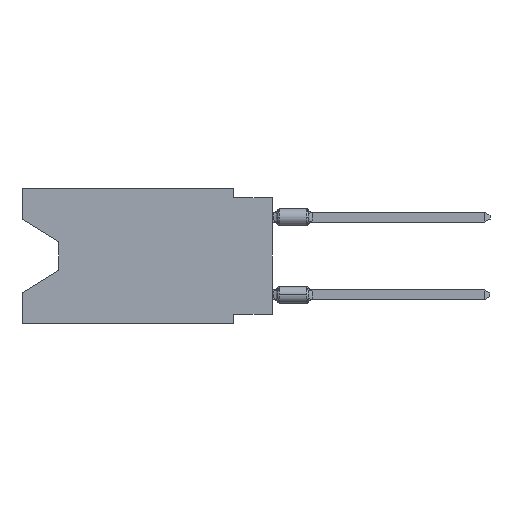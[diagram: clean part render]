
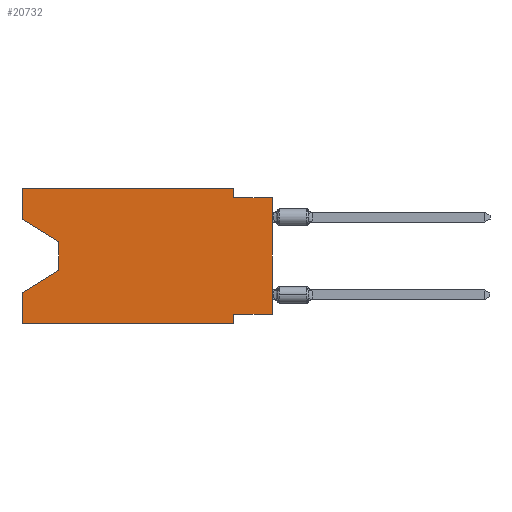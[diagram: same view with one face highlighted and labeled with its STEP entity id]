
A CAD part, left-side view. The second image highlights one B-rep face of the part: STEP entity #20732.
In plain terms, the highlighted planar face has unit normal (-1, 0, 0).
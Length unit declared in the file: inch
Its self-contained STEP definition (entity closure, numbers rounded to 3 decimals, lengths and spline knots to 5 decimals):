
#226 = CARTESIAN_POINT ( 'NONE',  ( 0., 0.1, -0.35 ) ) ;
#318 = LINE ( 'NONE', #9425, #13869 ) ;
#330 = LINE ( 'NONE', #23256, #6526 ) ;
#856 = EDGE_CURVE ( 'NONE', #12084, #20970, #318, .T. ) ;
#1134 = ORIENTED_EDGE ( 'NONE', *, *, #16072, .T. ) ;
#1196 = VECTOR ( 'NONE', #19495, 39.37008 ) ;
#1309 = CARTESIAN_POINT ( 'NONE',  ( 0., 0.55, -0.212 ) ) ;
#1514 = VECTOR ( 'NONE', #25624, 39.37008 ) ;
#1597 = CARTESIAN_POINT ( 'NONE',  ( 0., 0.55, -0.138 ) ) ;
#2020 = ORIENTED_EDGE ( 'NONE', *, *, #13922, .F. ) ;
#2694 = VECTOR ( 'NONE', #11086, 39.37008 ) ;
#2891 = DIRECTION ( 'NONE',  ( 0., 0., 1. ) ) ;
#3900 = VECTOR ( 'NONE', #18165, 39.37008 ) ;
#4437 = ORIENTED_EDGE ( 'NONE', *, *, #6137, .T. ) ;
#4848 = LINE ( 'NONE', #226, #22585 ) ;
#4886 = VERTEX_POINT ( 'NONE', #15136 ) ;
#5047 = EDGE_CURVE ( 'NONE', #11551, #13880, #15594, .T. ) ;
#5419 = CARTESIAN_POINT ( 'NONE',  ( 0., 0.645, 0. ) ) ;
#5496 = EDGE_CURVE ( 'NONE', #18941, #4886, #27695, .T. ) ;
#6137 = EDGE_CURVE ( 'NONE', #6393, #21999, #13539, .T. ) ;
#6333 = EDGE_CURVE ( 'NONE', #18941, #14355, #8129, .T. ) ;
#6393 = VERTEX_POINT ( 'NONE', #12887 ) ;
#6526 = VECTOR ( 'NONE', #20440, 39.37008 ) ;
#8006 = DIRECTION ( 'NONE',  ( 1., 0., 0. ) ) ;
#8129 = LINE ( 'NONE', #10205, #13457 ) ;
#8265 = LINE ( 'NONE', #10797, #11280 ) ;
#8493 = ORIENTED_EDGE ( 'NONE', *, *, #8763, .F. ) ;
#8708 = LINE ( 'NONE', #29246, #2694 ) ;
#8763 = EDGE_CURVE ( 'NONE', #6393, #21837, #16499, .T. ) ;
#9338 = DIRECTION ( 'NONE',  ( 0., 0., -1. ) ) ;
#9425 = CARTESIAN_POINT ( 'NONE',  ( 0., 0.1, 0. ) ) ;
#9585 = VECTOR ( 'NONE', #29248, 39.37008 ) ;
#10205 = CARTESIAN_POINT ( 'NONE',  ( 0., 0.645, 0. ) ) ;
#10797 = CARTESIAN_POINT ( 'NONE',  ( 0., 0.645, 0. ) ) ;
#11086 = DIRECTION ( 'NONE',  ( 0., 0.855, -0.519 ) ) ;
#11280 = VECTOR ( 'NONE', #24644, 39.37008 ) ;
#11527 = CARTESIAN_POINT ( 'NONE',  ( 0., 0.1, -0.025 ) ) ;
#11551 = VERTEX_POINT ( 'NONE', #14159 ) ;
#12025 = VERTEX_POINT ( 'NONE', #12751 ) ;
#12084 = VERTEX_POINT ( 'NONE', #19591 ) ;
#12751 = CARTESIAN_POINT ( 'NONE',  ( 0., 0., -0.025 ) ) ;
#12887 = CARTESIAN_POINT ( 'NONE',  ( 0., 0.645, -0.08025 ) ) ;
#13457 = VECTOR ( 'NONE', #28507, 39.37008 ) ;
#13539 = LINE ( 'NONE', #24712, #3900 ) ;
#13677 = ORIENTED_EDGE ( 'NONE', *, *, #27982, .F. ) ;
#13869 = VECTOR ( 'NONE', #18527, 39.37008 ) ;
#13880 = VERTEX_POINT ( 'NONE', #24006 ) ;
#13922 = EDGE_CURVE ( 'NONE', #20970, #12025, #26129, .T. ) ;
#14159 = CARTESIAN_POINT ( 'NONE',  ( 0., 0., -0.325 ) ) ;
#14355 = VERTEX_POINT ( 'NONE', #19683 ) ;
#14994 = FACE_OUTER_BOUND ( 'NONE', #23796, .T. ) ;
#15136 = CARTESIAN_POINT ( 'NONE',  ( 0., 0.1, -0.35 ) ) ;
#15162 = ORIENTED_EDGE ( 'NONE', *, *, #28124, .T. ) ;
#15594 = LINE ( 'NONE', #24775, #9585 ) ;
#16044 = VECTOR ( 'NONE', #19580, 39.37008 ) ;
#16072 = EDGE_CURVE ( 'NONE', #21999, #29130, #23784, .T. ) ;
#16265 = CARTESIAN_POINT ( 'NONE',  ( 0., 0.645, -0.35 ) ) ;
#16290 = EDGE_CURVE ( 'NONE', #13880, #4886, #4848, .T. ) ;
#16499 = LINE ( 'NONE', #5419, #20470 ) ;
#17390 = CARTESIAN_POINT ( 'NONE',  ( 0., 0.55, -0.138 ) ) ;
#17677 = PLANE ( 'NONE',  #22752 ) ;
#17972 = ORIENTED_EDGE ( 'NONE', *, *, #6333, .F. ) ;
#18165 = DIRECTION ( 'NONE',  ( 0., -0.855, -0.519 ) ) ;
#18527 = DIRECTION ( 'NONE',  ( 0., 0., -1. ) ) ;
#18941 = VERTEX_POINT ( 'NONE', #21852 ) ;
#19005 = ORIENTED_EDGE ( 'NONE', *, *, #856, .F. ) ;
#19495 = DIRECTION ( 'NONE',  ( 0., 0., -1. ) ) ;
#19580 = DIRECTION ( 'NONE',  ( 0., -1., 0. ) ) ;
#19591 = CARTESIAN_POINT ( 'NONE',  ( 0., 0.1, 0. ) ) ;
#19683 = CARTESIAN_POINT ( 'NONE',  ( 0., 0.645, -0.26975 ) ) ;
#19812 = ORIENTED_EDGE ( 'NONE', *, *, #5047, .F. ) ;
#20440 = DIRECTION ( 'NONE',  ( 0., 0., 1. ) ) ;
#20470 = VECTOR ( 'NONE', #2891, 39.37008 ) ;
#20732 = ADVANCED_FACE ( 'NONE', ( #14994 ), #17677, .F. ) ;
#20970 = VERTEX_POINT ( 'NONE', #11527 ) ;
#21837 = VERTEX_POINT ( 'NONE', #28209 ) ;
#21852 = CARTESIAN_POINT ( 'NONE',  ( 0., 0.645, -0.35 ) ) ;
#21958 = CARTESIAN_POINT ( 'NONE',  ( 0., 0.645, 0. ) ) ;
#21999 = VERTEX_POINT ( 'NONE', #17390 ) ;
#22585 = VECTOR ( 'NONE', #9338, 39.37008 ) ;
#22752 = AXIS2_PLACEMENT_3D ( 'NONE', #21958, #8006, #24206 ) ;
#23256 = CARTESIAN_POINT ( 'NONE',  ( 0., 0., 0. ) ) ;
#23784 = LINE ( 'NONE', #1597, #1196 ) ;
#23796 = EDGE_LOOP ( 'NONE', ( #4437, #1134, #28269, #17972, #24528, #26965, #19812, #15162, #2020, #19005, #13677, #8493 ) ) ;
#24006 = CARTESIAN_POINT ( 'NONE',  ( 0., 0.1, -0.325 ) ) ;
#24206 = DIRECTION ( 'NONE',  ( 0., 0., -1. ) ) ;
#24528 = ORIENTED_EDGE ( 'NONE', *, *, #5496, .T. ) ;
#24644 = DIRECTION ( 'NONE',  ( 0., -1., 0. ) ) ;
#24712 = CARTESIAN_POINT ( 'NONE',  ( 0., 0.645, -0.08025 ) ) ;
#24775 = CARTESIAN_POINT ( 'NONE',  ( 0., 0., -0.325 ) ) ;
#25624 = DIRECTION ( 'NONE',  ( 0., -1., 0. ) ) ;
#26129 = LINE ( 'NONE', #26578, #16044 ) ;
#26578 = CARTESIAN_POINT ( 'NONE',  ( 0., 0., -0.025 ) ) ;
#26965 = ORIENTED_EDGE ( 'NONE', *, *, #16290, .F. ) ;
#27695 = LINE ( 'NONE', #16265, #1514 ) ;
#27963 = EDGE_CURVE ( 'NONE', #29130, #14355, #8708, .T. ) ;
#27982 = EDGE_CURVE ( 'NONE', #21837, #12084, #8265, .T. ) ;
#28124 = EDGE_CURVE ( 'NONE', #11551, #12025, #330, .T. ) ;
#28209 = CARTESIAN_POINT ( 'NONE',  ( 0., 0.645, 0. ) ) ;
#28269 = ORIENTED_EDGE ( 'NONE', *, *, #27963, .T. ) ;
#28507 = DIRECTION ( 'NONE',  ( 0., 0., 1. ) ) ;
#29130 = VERTEX_POINT ( 'NONE', #1309 ) ;
#29246 = CARTESIAN_POINT ( 'NONE',  ( 0., 0.55, -0.212 ) ) ;
#29248 = DIRECTION ( 'NONE',  ( 0., 1., 0. ) ) ;
